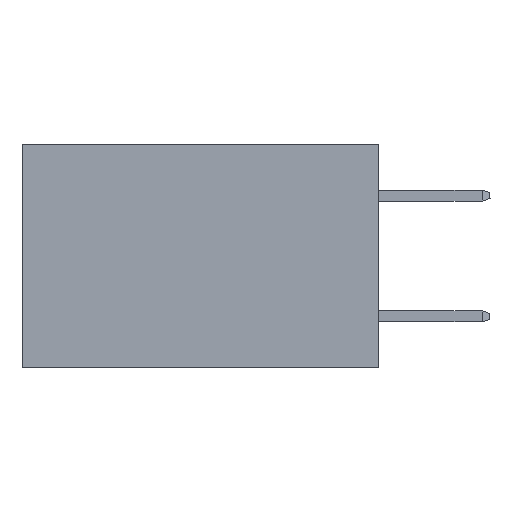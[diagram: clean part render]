
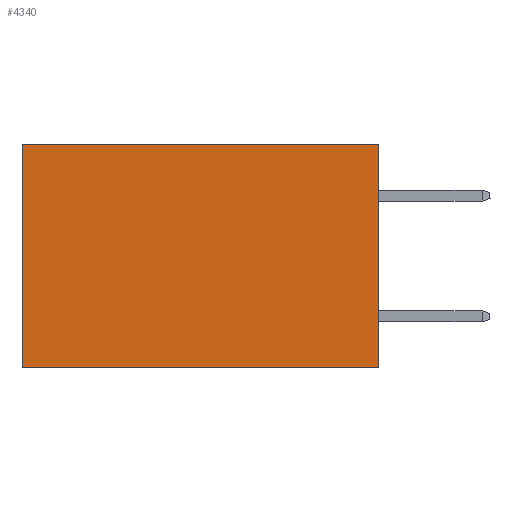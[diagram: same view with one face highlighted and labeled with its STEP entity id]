
A CAD part, left-side view. The second image highlights one B-rep face of the part: STEP entity #4340.
In plain terms, the highlighted planar face has unit normal (-1, 0, 0).
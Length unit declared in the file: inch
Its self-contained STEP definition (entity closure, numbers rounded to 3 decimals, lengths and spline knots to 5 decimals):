
#319 = DIRECTION ( 'NONE',  ( 0., 0., -1. ) ) ;
#380 = CARTESIAN_POINT ( 'NONE',  ( 0.277, 0.59, -0.37 ) ) ;
#899 = LINE ( 'NONE', #380, #16125 ) ;
#1422 = VECTOR ( 'NONE', #16289, 39.37008 ) ;
#1985 = ORIENTED_EDGE ( 'NONE', *, *, #6218, .T. ) ;
#2677 = AXIS2_PLACEMENT_3D ( 'NONE', #17582, #9202, #9102 ) ;
#3206 = CARTESIAN_POINT ( 'NONE',  ( 0.277, 0., -0.37 ) ) ;
#4340 = ADVANCED_FACE ( 'NONE', ( #14895 ), #8176, .F. ) ;
#4538 = CARTESIAN_POINT ( 'NONE',  ( 0.277, 0., 0. ) ) ;
#4719 = CARTESIAN_POINT ( 'NONE',  ( 0.277, 0., -0.37 ) ) ;
#4846 = CARTESIAN_POINT ( 'NONE',  ( 0.277, 0., -0.37 ) ) ;
#5588 = LINE ( 'NONE', #16329, #1422 ) ;
#5836 = EDGE_CURVE ( 'NONE', #10080, #13633, #5588, .T. ) ;
#6218 = EDGE_CURVE ( 'NONE', #13633, #11215, #899, .T. ) ;
#6310 = DIRECTION ( 'NONE',  ( 0., 0., -1. ) ) ;
#6319 = VECTOR ( 'NONE', #6310, 39.37008 ) ;
#8176 = PLANE ( 'NONE',  #2677 ) ;
#9102 = DIRECTION ( 'NONE',  ( 0., 0., -1. ) ) ;
#9202 = DIRECTION ( 'NONE',  ( 1., 0., 0. ) ) ;
#9238 = EDGE_CURVE ( 'NONE', #10080, #11178, #13964, .T. ) ;
#9248 = CARTESIAN_POINT ( 'NONE',  ( 0.277, 0.59, 0. ) ) ;
#9372 = LINE ( 'NONE', #4846, #16339 ) ;
#10080 = VERTEX_POINT ( 'NONE', #4538 ) ;
#10639 = EDGE_LOOP ( 'NONE', ( #1985, #17971, #14663, #18402 ) ) ;
#11178 = VERTEX_POINT ( 'NONE', #4719 ) ;
#11215 = VERTEX_POINT ( 'NONE', #14896 ) ;
#12007 = EDGE_CURVE ( 'NONE', #11178, #11215, #9372, .T. ) ;
#13633 = VERTEX_POINT ( 'NONE', #9248 ) ;
#13964 = LINE ( 'NONE', #3206, #6319 ) ;
#14663 = ORIENTED_EDGE ( 'NONE', *, *, #9238, .F. ) ;
#14895 = FACE_OUTER_BOUND ( 'NONE', #10639, .T. ) ;
#14896 = CARTESIAN_POINT ( 'NONE',  ( 0.277, 0.59, -0.37 ) ) ;
#16125 = VECTOR ( 'NONE', #319, 39.37008 ) ;
#16289 = DIRECTION ( 'NONE',  ( 0., 1., 0. ) ) ;
#16329 = CARTESIAN_POINT ( 'NONE',  ( 0.277, 0., 0. ) ) ;
#16339 = VECTOR ( 'NONE', #16370, 39.37008 ) ;
#16370 = DIRECTION ( 'NONE',  ( 0., 1., 0. ) ) ;
#17582 = CARTESIAN_POINT ( 'NONE',  ( 0.277, 0., -0.37 ) ) ;
#17971 = ORIENTED_EDGE ( 'NONE', *, *, #12007, .F. ) ;
#18402 = ORIENTED_EDGE ( 'NONE', *, *, #5836, .T. ) ;
